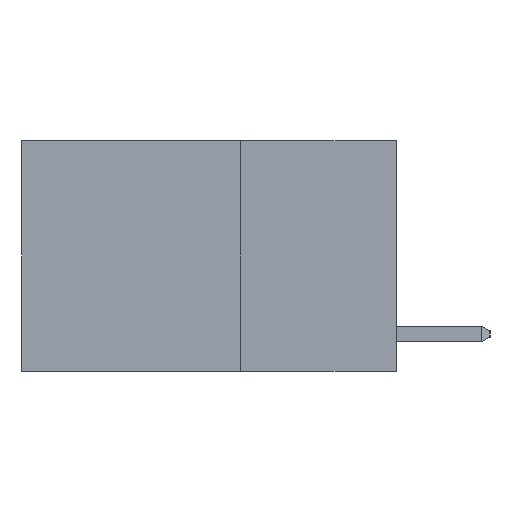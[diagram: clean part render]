
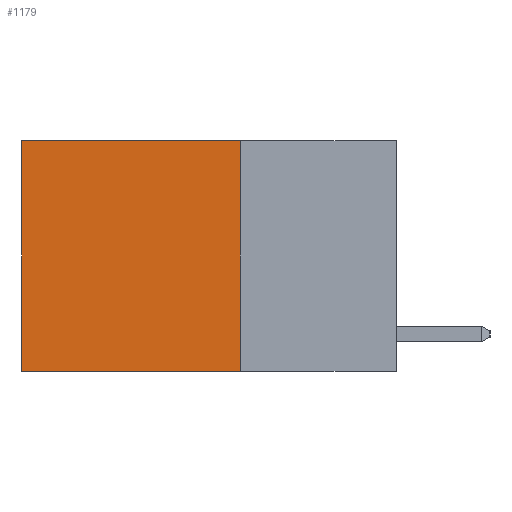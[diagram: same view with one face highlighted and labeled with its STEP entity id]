
A CAD part, left-side view. The second image highlights one B-rep face of the part: STEP entity #1179.
In plain terms, the highlighted planar face has unit normal (-1, 0, 0).
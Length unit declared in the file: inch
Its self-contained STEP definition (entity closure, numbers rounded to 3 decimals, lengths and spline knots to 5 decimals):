
#208 = EDGE_CURVE ( 'NONE', #941, #2005, #3798, .T. ) ;
#209 = ORIENTED_EDGE ( 'NONE', *, *, #7989, .F. ) ;
#242 = ORIENTED_EDGE ( 'NONE', *, *, #3011, .F. ) ;
#482 = ORIENTED_EDGE ( 'NONE', *, *, #6883, .T. ) ;
#567 = CARTESIAN_POINT ( 'NONE',  ( 0.2625, 0.25, 0. ) ) ;
#584 = VERTEX_POINT ( 'NONE', #7116 ) ;
#941 = VERTEX_POINT ( 'NONE', #6955 ) ;
#1005 = CARTESIAN_POINT ( 'NONE',  ( 0.2625, 0.6, 0. ) ) ;
#1179 = ADVANCED_FACE ( 'NONE', ( #8916 ), #3585, .F. ) ;
#1542 = DIRECTION ( 'NONE',  ( 0., 1., 0. ) ) ;
#2005 = VERTEX_POINT ( 'NONE', #7863 ) ;
#2163 = DIRECTION ( 'NONE',  ( 1., 0., 0. ) ) ;
#2731 = LINE ( 'NONE', #7322, #7909 ) ;
#3011 = EDGE_CURVE ( 'NONE', #3044, #584, #5036, .T. ) ;
#3017 = EDGE_LOOP ( 'NONE', ( #8051, #209, #242, #482 ) ) ;
#3044 = VERTEX_POINT ( 'NONE', #5582 ) ;
#3072 = VECTOR ( 'NONE', #1542, 39.37008 ) ;
#3094 = AXIS2_PLACEMENT_3D ( 'NONE', #567, #2163, #6974 ) ;
#3294 = DIRECTION ( 'NONE',  ( 0., 1., 0. ) ) ;
#3585 = PLANE ( 'NONE',  #3094 ) ;
#3690 = CARTESIAN_POINT ( 'NONE',  ( 0.2625, 0.25, -0.37 ) ) ;
#3798 = LINE ( 'NONE', #1005, #5573 ) ;
#4887 = CARTESIAN_POINT ( 'NONE',  ( 0.2625, 0.25, 0. ) ) ;
#4892 = LINE ( 'NONE', #3690, #3072 ) ;
#5036 = LINE ( 'NONE', #4887, #7050 ) ;
#5550 = DIRECTION ( 'NONE',  ( 0., 0., -1. ) ) ;
#5573 = VECTOR ( 'NONE', #6855, 39.37008 ) ;
#5582 = CARTESIAN_POINT ( 'NONE',  ( 0.2625, 0.25, 0. ) ) ;
#6855 = DIRECTION ( 'NONE',  ( 0., 0., -1. ) ) ;
#6883 = EDGE_CURVE ( 'NONE', #3044, #941, #2731, .T. ) ;
#6955 = CARTESIAN_POINT ( 'NONE',  ( 0.2625, 0.6, 0. ) ) ;
#6974 = DIRECTION ( 'NONE',  ( 0., 0., -1. ) ) ;
#7050 = VECTOR ( 'NONE', #5550, 39.37008 ) ;
#7116 = CARTESIAN_POINT ( 'NONE',  ( 0.2625, 0.25, -0.37 ) ) ;
#7322 = CARTESIAN_POINT ( 'NONE',  ( 0.2625, 0.25, 0. ) ) ;
#7863 = CARTESIAN_POINT ( 'NONE',  ( 0.2625, 0.6, -0.37 ) ) ;
#7909 = VECTOR ( 'NONE', #3294, 39.37008 ) ;
#7989 = EDGE_CURVE ( 'NONE', #584, #2005, #4892, .T. ) ;
#8051 = ORIENTED_EDGE ( 'NONE', *, *, #208, .T. ) ;
#8916 = FACE_OUTER_BOUND ( 'NONE', #3017, .T. ) ;
